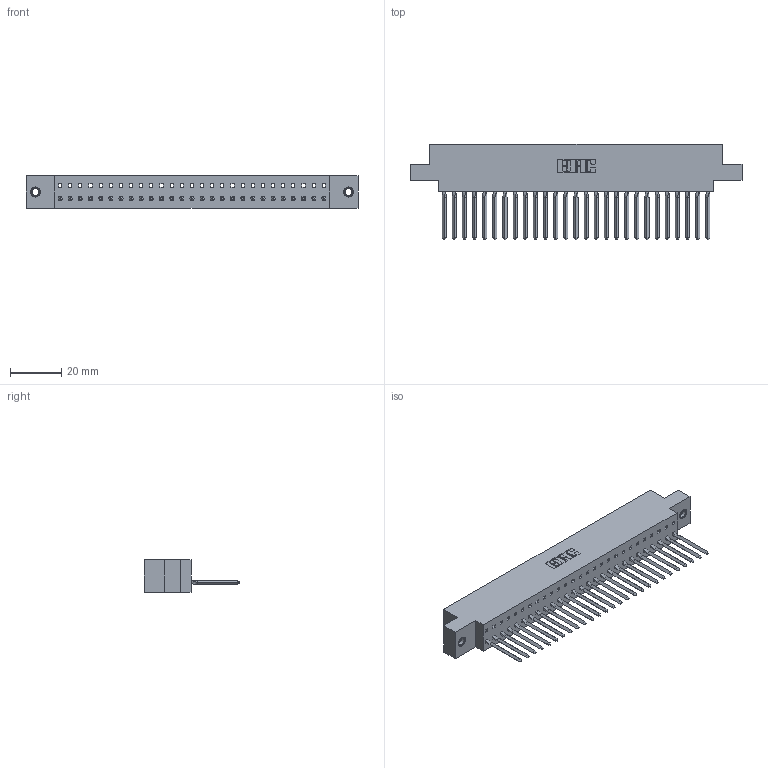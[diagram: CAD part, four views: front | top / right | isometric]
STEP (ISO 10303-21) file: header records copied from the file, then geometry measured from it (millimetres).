
FILE_DESCRIPTION (( 'STEP AP203' ), '1' );
FILE_NAME ('317-027-542-607.STEP', '2020-02-27T19:09:17', ( '' ), ( '' ), 'SwSTEP 2.0', 'SolidWorks 2016', '' );
FILE_SCHEMA (( 'CONFIG_CONTROL_DESIGN' ));
Length unit declared in the file: inch
Products named in the file (4): 317 Part_.156 Dia - TI; 345-250-001_345-250-005-103; 317-290-003_542; 317-027-542-607
Assembly tree (30 placements, depth 2):
  317-027-542-607
    317 Part_.156 Dia - TI
    317-290-003_542  x27
    345-250-001_345-250-005-103  x2
Bounding box: 129.69 x 37.34 x 12.7 mm (x, y, z)
Volume: 19621.6 mm3; surface area: 23635.9 mm2
Topology: 30 solids, 30 shells, 2187 faces, 6270 edges, 4046 vertices
Faces by surface type: plane 1818, cylinder 245, bspline 108, cone 12, torus 4
Entity records: 40460 total; most frequent: CARTESIAN_POINT 7401, ORIENTED_EDGE 7084, DIRECTION 5970, EDGE_CURVE 3542, LINE 3352, VECTOR 3352, VERTEX_POINT 2352, AXIS2_PLACEMENT_3D 1309
